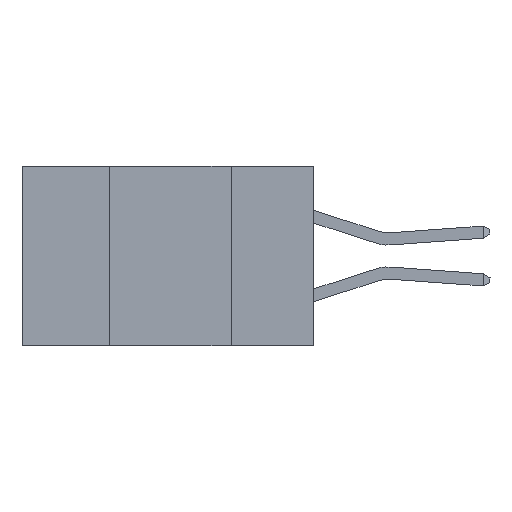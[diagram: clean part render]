
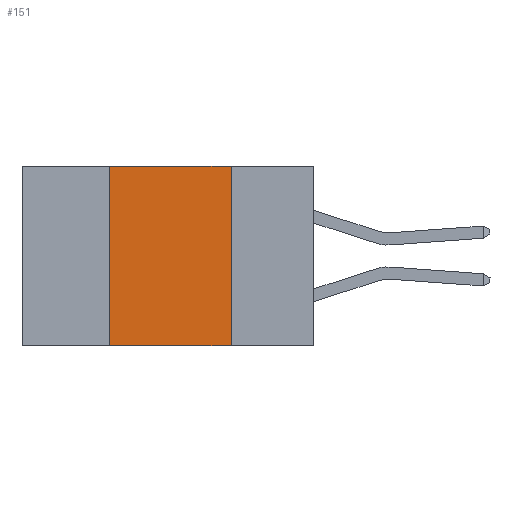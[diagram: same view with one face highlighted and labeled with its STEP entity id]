
A CAD part, left-side view. The second image highlights one B-rep face of the part: STEP entity #151.
In plain terms, the highlighted planar face has unit normal (-1, 0, 0).
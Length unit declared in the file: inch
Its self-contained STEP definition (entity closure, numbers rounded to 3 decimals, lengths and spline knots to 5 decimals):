
#151 = ADVANCED_FACE ( 'NONE', ( #10887 ), #2264, .F. ) ;
#938 = AXIS2_PLACEMENT_3D ( 'NONE', #2255, #2240, #2189 ) ;
#1044 = CARTESIAN_POINT ( 'NONE',  ( 0., 0.17, 0. ) ) ;
#1864 = LINE ( 'NONE', #1044, #12079 ) ;
#1981 = LINE ( 'NONE', #3104, #12169 ) ;
#2100 = VECTOR ( 'NONE', #10969, 39.37008 ) ;
#2189 = DIRECTION ( 'NONE',  ( 0., 0., -1. ) ) ;
#2240 = DIRECTION ( 'NONE',  ( 1., 0., 0. ) ) ;
#2255 = CARTESIAN_POINT ( 'NONE',  ( 0., 0.6, 0. ) ) ;
#2264 = PLANE ( 'NONE',  #938 ) ;
#2657 = CARTESIAN_POINT ( 'NONE',  ( 0., 0.17, -0.37 ) ) ;
#2870 = CARTESIAN_POINT ( 'NONE',  ( 0., 0.42, 0. ) ) ;
#3104 = CARTESIAN_POINT ( 'NONE',  ( 0., 0.6, -0.37 ) ) ;
#3407 = DIRECTION ( 'NONE',  ( 0., 0., -1. ) ) ;
#4214 = ORIENTED_EDGE ( 'NONE', *, *, #6205, .F. ) ;
#4937 = LINE ( 'NONE', #7092, #2100 ) ;
#5254 = DIRECTION ( 'NONE',  ( 0., -1., 0. ) ) ;
#5359 = ORIENTED_EDGE ( 'NONE', *, *, #11551, .F. ) ;
#6098 = CARTESIAN_POINT ( 'NONE',  ( 0., 0.42, -0.37 ) ) ;
#6205 = EDGE_CURVE ( 'NONE', #10149, #7037, #1864, .T. ) ;
#7037 = VERTEX_POINT ( 'NONE', #2657 ) ;
#7092 = CARTESIAN_POINT ( 'NONE',  ( 0., 0.42, 0. ) ) ;
#7240 = CARTESIAN_POINT ( 'NONE',  ( 0., 0.6, 0. ) ) ;
#7535 = CARTESIAN_POINT ( 'NONE',  ( 0., 0.17, 0. ) ) ;
#7629 = ORIENTED_EDGE ( 'NONE', *, *, #8112, .T. ) ;
#8112 = EDGE_CURVE ( 'NONE', #12078, #7037, #1981, .T. ) ;
#9336 = LINE ( 'NONE', #7240, #11805 ) ;
#9742 = ORIENTED_EDGE ( 'NONE', *, *, #9981, .F. ) ;
#9981 = EDGE_CURVE ( 'NONE', #12078, #10811, #4937, .T. ) ;
#10149 = VERTEX_POINT ( 'NONE', #7535 ) ;
#10434 = EDGE_LOOP ( 'NONE', ( #4214, #5359, #9742, #7629 ) ) ;
#10811 = VERTEX_POINT ( 'NONE', #2870 ) ;
#10887 = FACE_OUTER_BOUND ( 'NONE', #10434, .T. ) ;
#10969 = DIRECTION ( 'NONE',  ( 0., 0., 1. ) ) ;
#11551 = EDGE_CURVE ( 'NONE', #10811, #10149, #9336, .T. ) ;
#11805 = VECTOR ( 'NONE', #5254, 39.37008 ) ;
#11918 = DIRECTION ( 'NONE',  ( 0., -1., 0. ) ) ;
#12078 = VERTEX_POINT ( 'NONE', #6098 ) ;
#12079 = VECTOR ( 'NONE', #3407, 39.37008 ) ;
#12169 = VECTOR ( 'NONE', #11918, 39.37008 ) ;
